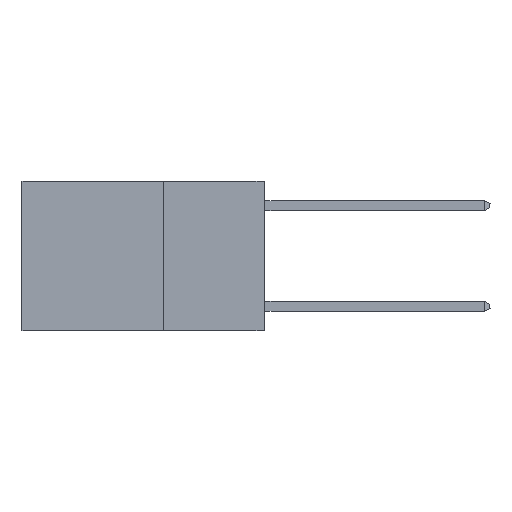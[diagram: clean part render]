
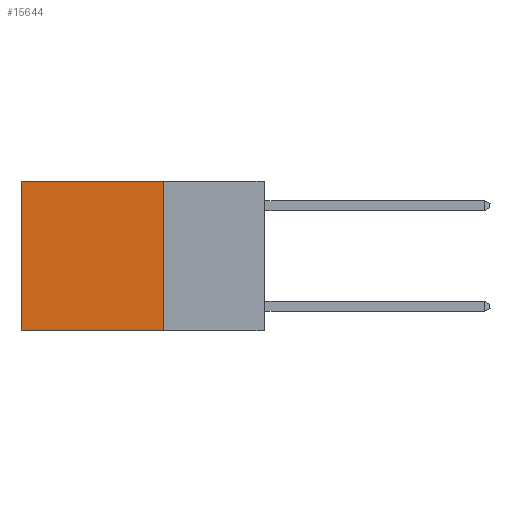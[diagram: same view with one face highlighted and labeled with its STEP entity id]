
A CAD part, left-side view. The second image highlights one B-rep face of the part: STEP entity #15644.
In plain terms, the highlighted planar face has unit normal (-1, 0, 0).
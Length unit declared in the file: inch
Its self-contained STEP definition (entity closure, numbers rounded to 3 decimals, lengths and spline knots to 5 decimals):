
#578 = ORIENTED_EDGE ( 'NONE', *, *, #6877, .T. ) ;
#682 = VERTEX_POINT ( 'NONE', #20953 ) ;
#708 = EDGE_CURVE ( 'NONE', #682, #11232, #14393, .T. ) ;
#955 = CARTESIAN_POINT ( 'NONE',  ( 0.2625, 0.25, -0.37 ) ) ;
#2309 = CARTESIAN_POINT ( 'NONE',  ( 0.2625, 0.25, 0. ) ) ;
#2358 = VECTOR ( 'NONE', #8125, 39.37008 ) ;
#2677 = CARTESIAN_POINT ( 'NONE',  ( 0.2625, 0.6, -0.37 ) ) ;
#2771 = CARTESIAN_POINT ( 'NONE',  ( 0.2625, 0.25, 0. ) ) ;
#2869 = EDGE_CURVE ( 'NONE', #682, #16560, #3181, .T. ) ;
#3181 = LINE ( 'NONE', #10135, #2358 ) ;
#4060 = LINE ( 'NONE', #12657, #15925 ) ;
#5985 = AXIS2_PLACEMENT_3D ( 'NONE', #2771, #9488, #16378 ) ;
#6877 = EDGE_CURVE ( 'NONE', #11232, #20586, #4060, .T. ) ;
#7415 = ORIENTED_EDGE ( 'NONE', *, *, #2869, .F. ) ;
#8039 = PLANE ( 'NONE',  #5985 ) ;
#8125 = DIRECTION ( 'NONE',  ( 0., 0., -1. ) ) ;
#9488 = DIRECTION ( 'NONE',  ( 1., 0., 0. ) ) ;
#9580 = CARTESIAN_POINT ( 'NONE',  ( 0.2625, 0.6, 0. ) ) ;
#9595 = FACE_OUTER_BOUND ( 'NONE', #16877, .T. ) ;
#9785 = EDGE_CURVE ( 'NONE', #16560, #20586, #16403, .T. ) ;
#10135 = CARTESIAN_POINT ( 'NONE',  ( 0.2625, 0.25, 0. ) ) ;
#11166 = DIRECTION ( 'NONE',  ( 0., 1., 0. ) ) ;
#11232 = VERTEX_POINT ( 'NONE', #9580 ) ;
#11864 = VECTOR ( 'NONE', #19293, 39.37008 ) ;
#12657 = CARTESIAN_POINT ( 'NONE',  ( 0.2625, 0.6, 0. ) ) ;
#12873 = DIRECTION ( 'NONE',  ( 0., 0., -1. ) ) ;
#14393 = LINE ( 'NONE', #2309, #11864 ) ;
#14437 = CARTESIAN_POINT ( 'NONE',  ( 0.2625, 0.25, -0.37 ) ) ;
#15644 = ADVANCED_FACE ( 'NONE', ( #9595 ), #8039, .F. ) ;
#15925 = VECTOR ( 'NONE', #12873, 39.37008 ) ;
#16378 = DIRECTION ( 'NONE',  ( 0., 0., -1. ) ) ;
#16403 = LINE ( 'NONE', #14437, #20911 ) ;
#16560 = VERTEX_POINT ( 'NONE', #955 ) ;
#16877 = EDGE_LOOP ( 'NONE', ( #578, #17104, #7415, #17798 ) ) ;
#17104 = ORIENTED_EDGE ( 'NONE', *, *, #9785, .F. ) ;
#17798 = ORIENTED_EDGE ( 'NONE', *, *, #708, .T. ) ;
#19293 = DIRECTION ( 'NONE',  ( 0., 1., 0. ) ) ;
#20586 = VERTEX_POINT ( 'NONE', #2677 ) ;
#20911 = VECTOR ( 'NONE', #11166, 39.37008 ) ;
#20953 = CARTESIAN_POINT ( 'NONE',  ( 0.2625, 0.25, 0. ) ) ;
